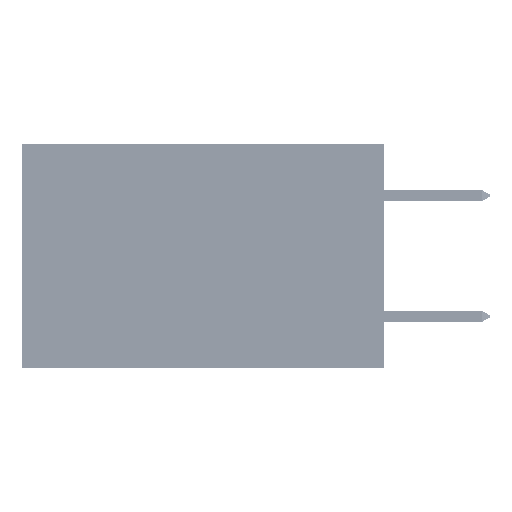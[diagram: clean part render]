
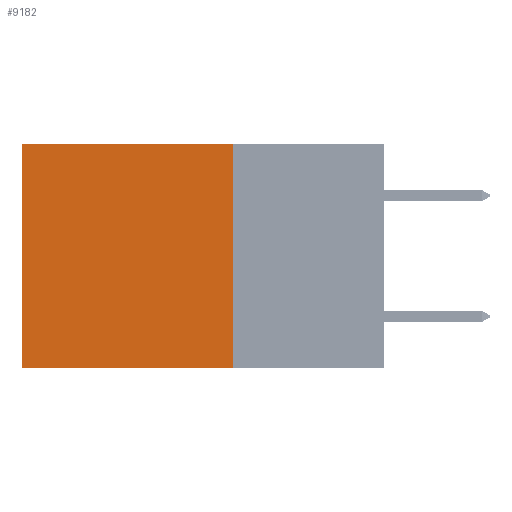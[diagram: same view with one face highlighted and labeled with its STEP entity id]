
A CAD part, left-side view. The second image highlights one B-rep face of the part: STEP entity #9182.
In plain terms, the highlighted planar face has unit normal (-1, 0, 0).
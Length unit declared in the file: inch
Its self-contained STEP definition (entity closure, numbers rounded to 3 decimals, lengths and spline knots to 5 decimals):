
#69 = VERTEX_POINT ( 'NONE', #16185 ) ;
#6782 = AXIS2_PLACEMENT_3D ( 'NONE', #10594, #14793, #38796 ) ;
#6985 = DIRECTION ( 'NONE',  ( 0., 1., 0. ) ) ;
#8351 = VECTOR ( 'NONE', #37370, 39.37008 ) ;
#9182 = ADVANCED_FACE ( 'NONE', ( #47946 ), #18869, .F. ) ;
#10594 = CARTESIAN_POINT ( 'NONE',  ( 0.2875, 0.25, 0. ) ) ;
#13781 = DIRECTION ( 'NONE',  ( 0., 0., -1. ) ) ;
#14793 = DIRECTION ( 'NONE',  ( 1., 0., 0. ) ) ;
#14885 = CARTESIAN_POINT ( 'NONE',  ( 0.2875, 0.25, 0. ) ) ;
#15028 = LINE ( 'NONE', #14885, #24489 ) ;
#15860 = VERTEX_POINT ( 'NONE', #51282 ) ;
#16185 = CARTESIAN_POINT ( 'NONE',  ( 0.2875, 0.25, 0. ) ) ;
#16403 = VECTOR ( 'NONE', #13781, 39.37008 ) ;
#17640 = DIRECTION ( 'NONE',  ( 0., 0., -1. ) ) ;
#18869 = PLANE ( 'NONE',  #6782 ) ;
#18961 = LINE ( 'NONE', #37454, #16403 ) ;
#19077 = LINE ( 'NONE', #29325, #8351 ) ;
#22044 = CARTESIAN_POINT ( 'NONE',  ( 0.2875, 0.25, 0. ) ) ;
#24489 = VECTOR ( 'NONE', #6985, 39.37008 ) ;
#24873 = EDGE_CURVE ( 'NONE', #15860, #25093, #18961, .T. ) ;
#25093 = VERTEX_POINT ( 'NONE', #37970 ) ;
#29325 = CARTESIAN_POINT ( 'NONE',  ( 0.2875, 0.25, -0.37 ) ) ;
#35862 = ORIENTED_EDGE ( 'NONE', *, *, #36411, .T. ) ;
#36411 = EDGE_CURVE ( 'NONE', #69, #15860, #15028, .T. ) ;
#37370 = DIRECTION ( 'NONE',  ( 0., 1., 0. ) ) ;
#37454 = CARTESIAN_POINT ( 'NONE',  ( 0.2875, 0.6, 0. ) ) ;
#37970 = CARTESIAN_POINT ( 'NONE',  ( 0.2875, 0.6, -0.37 ) ) ;
#38131 = ORIENTED_EDGE ( 'NONE', *, *, #24873, .T. ) ;
#38620 = VERTEX_POINT ( 'NONE', #38706 ) ;
#38706 = CARTESIAN_POINT ( 'NONE',  ( 0.2875, 0.25, -0.37 ) ) ;
#38796 = DIRECTION ( 'NONE',  ( 0., 0., -1. ) ) ;
#39122 = EDGE_CURVE ( 'NONE', #69, #38620, #49833, .T. ) ;
#39818 = EDGE_CURVE ( 'NONE', #38620, #25093, #19077, .T. ) ;
#45444 = VECTOR ( 'NONE', #17640, 39.37008 ) ;
#46334 = EDGE_LOOP ( 'NONE', ( #38131, #47232, #51506, #35862 ) ) ;
#47232 = ORIENTED_EDGE ( 'NONE', *, *, #39818, .F. ) ;
#47946 = FACE_OUTER_BOUND ( 'NONE', #46334, .T. ) ;
#49833 = LINE ( 'NONE', #22044, #45444 ) ;
#51282 = CARTESIAN_POINT ( 'NONE',  ( 0.2875, 0.6, 0. ) ) ;
#51506 = ORIENTED_EDGE ( 'NONE', *, *, #39122, .F. ) ;
